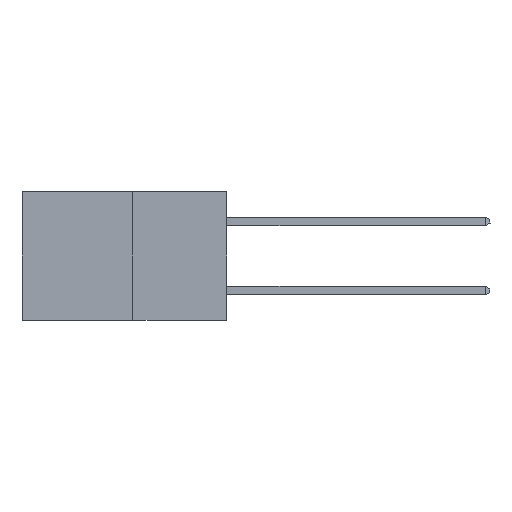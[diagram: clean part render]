
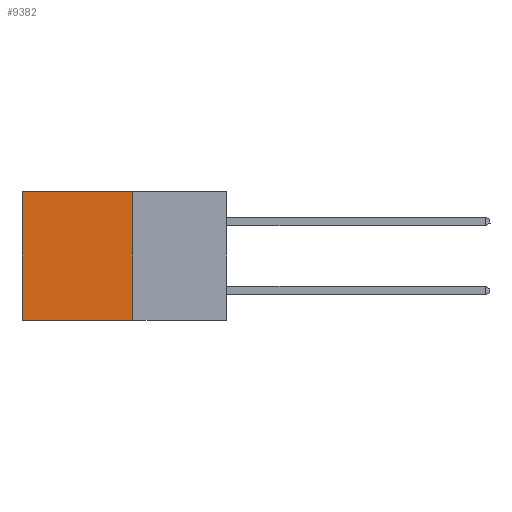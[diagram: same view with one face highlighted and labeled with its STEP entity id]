
A CAD part, left-side view. The second image highlights one B-rep face of the part: STEP entity #9382.
In plain terms, the highlighted planar face has unit normal (-1, 0, 0).
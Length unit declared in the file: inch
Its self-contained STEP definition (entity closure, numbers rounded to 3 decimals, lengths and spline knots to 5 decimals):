
#544 = ORIENTED_EDGE ( 'NONE', *, *, #4587, .F. ) ;
#699 = CARTESIAN_POINT ( 'NONE',  ( 0.277, 0.27, -0.37 ) ) ;
#929 = LINE ( 'NONE', #3730, #10351 ) ;
#1095 = VECTOR ( 'NONE', #6890, 39.37008 ) ;
#1350 = EDGE_CURVE ( 'NONE', #10298, #8380, #6008, .T. ) ;
#1729 = CARTESIAN_POINT ( 'NONE',  ( 0.277, 0.27, 0. ) ) ;
#1882 = PLANE ( 'NONE',  #7929 ) ;
#2690 = FACE_OUTER_BOUND ( 'NONE', #4930, .T. ) ;
#3087 = LINE ( 'NONE', #9561, #7204 ) ;
#3239 = DIRECTION ( 'NONE',  ( 0., 0., -1. ) ) ;
#3730 = CARTESIAN_POINT ( 'NONE',  ( 0.277, 0.59, -0.37 ) ) ;
#3767 = EDGE_CURVE ( 'NONE', #8380, #7900, #929, .T. ) ;
#3942 = CARTESIAN_POINT ( 'NONE',  ( 0.277, 0.59, 0. ) ) ;
#4009 = DIRECTION ( 'NONE',  ( 0., 0., -1. ) ) ;
#4587 = EDGE_CURVE ( 'NONE', #10298, #7329, #11212, .T. ) ;
#4930 = EDGE_LOOP ( 'NONE', ( #8917, #8823, #544, #8829 ) ) ;
#5168 = CARTESIAN_POINT ( 'NONE',  ( 0.277, 0.59, -0.37 ) ) ;
#5739 = VECTOR ( 'NONE', #10204, 39.37008 ) ;
#6008 = LINE ( 'NONE', #6096, #5739 ) ;
#6096 = CARTESIAN_POINT ( 'NONE',  ( 0.277, 0.27, 0. ) ) ;
#6158 = EDGE_CURVE ( 'NONE', #7329, #7900, #3087, .T. ) ;
#6595 = CARTESIAN_POINT ( 'NONE',  ( 0.277, 0.27, -0.37 ) ) ;
#6890 = DIRECTION ( 'NONE',  ( 0., 0., -1. ) ) ;
#7015 = CARTESIAN_POINT ( 'NONE',  ( 0.277, 0.27, -0.37 ) ) ;
#7204 = VECTOR ( 'NONE', #9389, 39.37008 ) ;
#7329 = VERTEX_POINT ( 'NONE', #6595 ) ;
#7900 = VERTEX_POINT ( 'NONE', #5168 ) ;
#7929 = AXIS2_PLACEMENT_3D ( 'NONE', #699, #9139, #4009 ) ;
#8380 = VERTEX_POINT ( 'NONE', #3942 ) ;
#8823 = ORIENTED_EDGE ( 'NONE', *, *, #6158, .F. ) ;
#8829 = ORIENTED_EDGE ( 'NONE', *, *, #1350, .T. ) ;
#8917 = ORIENTED_EDGE ( 'NONE', *, *, #3767, .T. ) ;
#9139 = DIRECTION ( 'NONE',  ( 1., 0., 0. ) ) ;
#9382 = ADVANCED_FACE ( 'NONE', ( #2690 ), #1882, .F. ) ;
#9389 = DIRECTION ( 'NONE',  ( 0., 1., 0. ) ) ;
#9561 = CARTESIAN_POINT ( 'NONE',  ( 0.277, 0.27, -0.37 ) ) ;
#10204 = DIRECTION ( 'NONE',  ( 0., 1., 0. ) ) ;
#10298 = VERTEX_POINT ( 'NONE', #1729 ) ;
#10351 = VECTOR ( 'NONE', #3239, 39.37008 ) ;
#11212 = LINE ( 'NONE', #7015, #1095 ) ;
